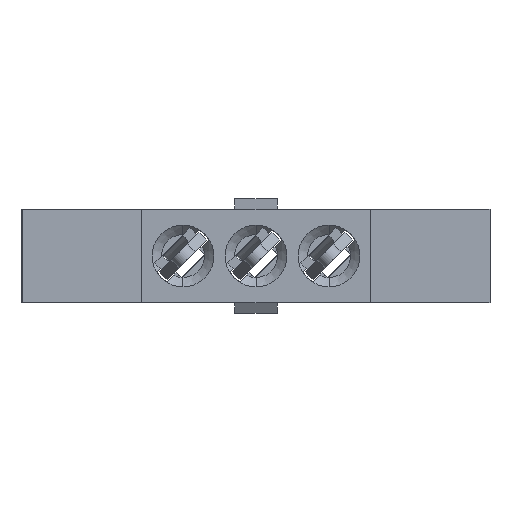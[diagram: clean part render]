
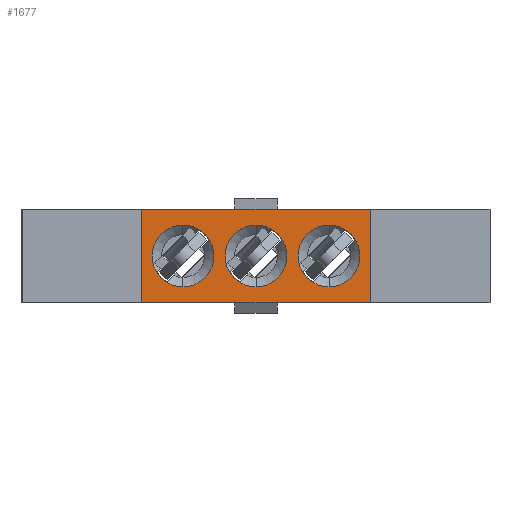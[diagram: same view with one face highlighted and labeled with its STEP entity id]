
A CAD part, front view. The second image highlights one B-rep face of the part: STEP entity #1677.
In plain terms, the highlighted planar face has unit normal (0, -1, 0).
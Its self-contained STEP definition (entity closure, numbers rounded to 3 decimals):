
#22 = DIRECTION ( 'NONE',  ( 0., 1., 0. ) ) ;
#100 = CARTESIAN_POINT ( 'NONE',  ( 7.925, -11.176, 0. ) ) ;
#134 = VERTEX_POINT ( 'NONE', #4937 ) ;
#208 = CARTESIAN_POINT ( 'NONE',  ( 0., -11.176, 0. ) ) ;
#235 = CIRCLE ( 'NONE', #864, 1.676 ) ;
#549 = EDGE_LOOP ( 'NONE', ( #6297, #2904 ) ) ;
#564 = CIRCLE ( 'NONE', #1767, 1.676 ) ;
#620 = CIRCLE ( 'NONE', #1384, 1.676 ) ;
#704 = EDGE_CURVE ( 'NONE', #2894, #1035, #717, .T. ) ;
#717 = LINE ( 'NONE', #6544, #2399 ) ;
#743 = EDGE_LOOP ( 'NONE', ( #883, #2566 ) ) ;
#845 = DIRECTION ( 'NONE',  ( 0., 0., 1. ) ) ;
#864 = AXIS2_PLACEMENT_3D ( 'NONE', #100, #3715, #2695 ) ;
#883 = ORIENTED_EDGE ( 'NONE', *, *, #4159, .T. ) ;
#1028 = CARTESIAN_POINT ( 'NONE',  ( 7.925, -11.176, 1.676 ) ) ;
#1035 = VERTEX_POINT ( 'NONE', #5929 ) ;
#1260 = CIRCLE ( 'NONE', #6158, 1.676 ) ;
#1333 = CARTESIAN_POINT ( 'NONE',  ( 7.925, -11.176, 0. ) ) ;
#1371 = VERTEX_POINT ( 'NONE', #3113 ) ;
#1384 = AXIS2_PLACEMENT_3D ( 'NONE', #5391, #6515, #845 ) ;
#1426 = FACE_OUTER_BOUND ( 'NONE', #2476, .T. ) ;
#1541 = DIRECTION ( 'NONE',  ( 0., 1., 0. ) ) ;
#1564 = ORIENTED_EDGE ( 'NONE', *, *, #2822, .T. ) ;
#1583 = ORIENTED_EDGE ( 'NONE', *, *, #704, .F. ) ;
#1649 = EDGE_CURVE ( 'NONE', #1371, #134, #4518, .T. ) ;
#1668 = CARTESIAN_POINT ( 'NONE',  ( -2.235, -11.176, -2.54 ) ) ;
#1677 = ADVANCED_FACE ( 'NONE', ( #4840, #6628, #3206, #1426 ), #5864, .F. ) ;
#1725 = EDGE_CURVE ( 'NONE', #4992, #6248, #2957, .T. ) ;
#1767 = AXIS2_PLACEMENT_3D ( 'NONE', #4345, #4866, #1836 ) ;
#1812 = LINE ( 'NONE', #6039, #2305 ) ;
#1836 = DIRECTION ( 'NONE',  ( 0., 0., 1. ) ) ;
#1896 = EDGE_CURVE ( 'NONE', #6248, #2894, #1812, .T. ) ;
#1901 = DIRECTION ( 'NONE',  ( 1., 0., 0. ) ) ;
#2071 = CARTESIAN_POINT ( 'NONE',  ( 3.962, -11.176, -1.676 ) ) ;
#2106 = VERTEX_POINT ( 'NONE', #2071 ) ;
#2154 = EDGE_LOOP ( 'NONE', ( #3794, #1564 ) ) ;
#2305 = VECTOR ( 'NONE', #1901, 1000. ) ;
#2337 = EDGE_CURVE ( 'NONE', #3234, #6090, #4344, .T. ) ;
#2340 = CARTESIAN_POINT ( 'NONE',  ( -2.235, -11.176, -2.54 ) ) ;
#2399 = VECTOR ( 'NONE', #3421, 1000. ) ;
#2476 = EDGE_LOOP ( 'NONE', ( #5883, #3900, #1583, #3518 ) ) ;
#2488 = VERTEX_POINT ( 'NONE', #6648 ) ;
#2562 = LINE ( 'NONE', #3753, #4851 ) ;
#2566 = ORIENTED_EDGE ( 'NONE', *, *, #1649, .T. ) ;
#2583 = DIRECTION ( 'NONE',  ( 0., 0., 1. ) ) ;
#2695 = DIRECTION ( 'NONE',  ( 0., 0., 1. ) ) ;
#2822 = EDGE_CURVE ( 'NONE', #2106, #2488, #1260, .T. ) ;
#2894 = VERTEX_POINT ( 'NONE', #4201 ) ;
#2897 = DIRECTION ( 'NONE',  ( 0., 0., 1. ) ) ;
#2904 = ORIENTED_EDGE ( 'NONE', *, *, #4547, .T. ) ;
#2957 = LINE ( 'NONE', #1668, #6456 ) ;
#3113 = CARTESIAN_POINT ( 'NONE',  ( 0., -11.176, -1.676 ) ) ;
#3158 = CARTESIAN_POINT ( 'NONE',  ( 3.962, -11.176, 0. ) ) ;
#3206 = FACE_BOUND ( 'NONE', #743, .T. ) ;
#3234 = VERTEX_POINT ( 'NONE', #1028 ) ;
#3421 = DIRECTION ( 'NONE',  ( 0., 0., -1. ) ) ;
#3518 = ORIENTED_EDGE ( 'NONE', *, *, #1896, .F. ) ;
#3617 = AXIS2_PLACEMENT_3D ( 'NONE', #1333, #6014, #2897 ) ;
#3639 = DIRECTION ( 'NONE',  ( 0., 0., 1. ) ) ;
#3715 = DIRECTION ( 'NONE',  ( 0., 1., 0. ) ) ;
#3753 = CARTESIAN_POINT ( 'NONE',  ( -2.235, -11.176, -2.54 ) ) ;
#3794 = ORIENTED_EDGE ( 'NONE', *, *, #5702, .T. ) ;
#3900 = ORIENTED_EDGE ( 'NONE', *, *, #4880, .F. ) ;
#4159 = EDGE_CURVE ( 'NONE', #134, #1371, #564, .T. ) ;
#4201 = CARTESIAN_POINT ( 'NONE',  ( 10.16, -11.176, 2.54 ) ) ;
#4278 = DIRECTION ( 'NONE',  ( -1., 0., 0. ) ) ;
#4344 = CIRCLE ( 'NONE', #3617, 1.676 ) ;
#4345 = CARTESIAN_POINT ( 'NONE',  ( 0., -11.176, 0. ) ) ;
#4472 = DIRECTION ( 'NONE',  ( 0., 1., 0. ) ) ;
#4518 = CIRCLE ( 'NONE', #6512, 1.676 ) ;
#4547 = EDGE_CURVE ( 'NONE', #6090, #3234, #235, .T. ) ;
#4788 = DIRECTION ( 'NONE',  ( 0., 0., 1. ) ) ;
#4807 = DIRECTION ( 'NONE',  ( 0., 0., 1. ) ) ;
#4840 = FACE_BOUND ( 'NONE', #549, .T. ) ;
#4851 = VECTOR ( 'NONE', #4278, 1000. ) ;
#4866 = DIRECTION ( 'NONE',  ( 0., 1., 0. ) ) ;
#4880 = EDGE_CURVE ( 'NONE', #1035, #4992, #2562, .T. ) ;
#4937 = CARTESIAN_POINT ( 'NONE',  ( 0., -11.176, 1.676 ) ) ;
#4992 = VERTEX_POINT ( 'NONE', #2340 ) ;
#5255 = CARTESIAN_POINT ( 'NONE',  ( 7.925, -11.176, -1.676 ) ) ;
#5391 = CARTESIAN_POINT ( 'NONE',  ( 3.962, -11.176, 0. ) ) ;
#5702 = EDGE_CURVE ( 'NONE', #2488, #2106, #620, .T. ) ;
#5715 = CARTESIAN_POINT ( 'NONE',  ( 0., -11.176, 0. ) ) ;
#5864 = PLANE ( 'NONE',  #6593 ) ;
#5883 = ORIENTED_EDGE ( 'NONE', *, *, #1725, .F. ) ;
#5929 = CARTESIAN_POINT ( 'NONE',  ( 10.16, -11.176, -2.54 ) ) ;
#6014 = DIRECTION ( 'NONE',  ( 0., 1., 0. ) ) ;
#6039 = CARTESIAN_POINT ( 'NONE',  ( -2.235, -11.176, 2.54 ) ) ;
#6090 = VERTEX_POINT ( 'NONE', #5255 ) ;
#6155 = CARTESIAN_POINT ( 'NONE',  ( -2.235, -11.176, 2.54 ) ) ;
#6158 = AXIS2_PLACEMENT_3D ( 'NONE', #3158, #1541, #2583 ) ;
#6248 = VERTEX_POINT ( 'NONE', #6155 ) ;
#6297 = ORIENTED_EDGE ( 'NONE', *, *, #2337, .T. ) ;
#6456 = VECTOR ( 'NONE', #4807, 1000. ) ;
#6512 = AXIS2_PLACEMENT_3D ( 'NONE', #5715, #22, #3639 ) ;
#6515 = DIRECTION ( 'NONE',  ( 0., 1., 0. ) ) ;
#6544 = CARTESIAN_POINT ( 'NONE',  ( 10.16, -11.176, -2.54 ) ) ;
#6593 = AXIS2_PLACEMENT_3D ( 'NONE', #208, #4472, #4788 ) ;
#6628 = FACE_BOUND ( 'NONE', #2154, .T. ) ;
#6648 = CARTESIAN_POINT ( 'NONE',  ( 3.962, -11.176, 1.676 ) ) ;
